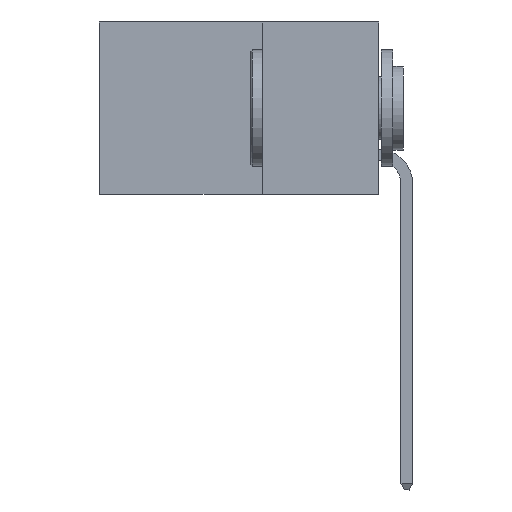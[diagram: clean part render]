
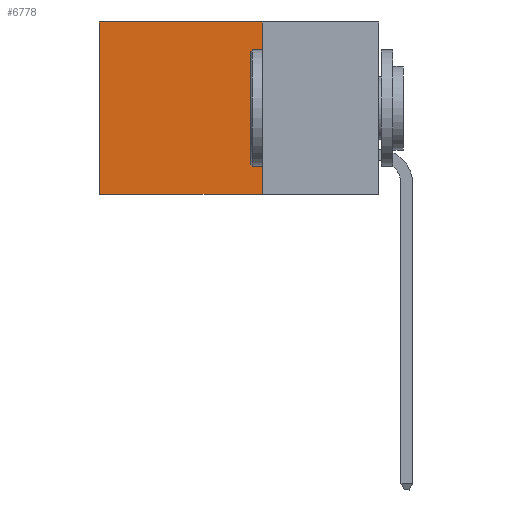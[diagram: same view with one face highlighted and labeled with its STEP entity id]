
A CAD part, left-side view. The second image highlights one B-rep face of the part: STEP entity #6778.
In plain terms, the highlighted planar face has unit normal (-1, 0, 0).
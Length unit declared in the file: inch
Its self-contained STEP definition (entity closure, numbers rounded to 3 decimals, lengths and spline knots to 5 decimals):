
#124 = LINE ( 'NONE', #7433, #5244 ) ;
#285 = VERTEX_POINT ( 'NONE', #12452 ) ;
#310 = CARTESIAN_POINT ( 'NONE',  ( 0.298, 0.25, -0.37 ) ) ;
#1391 = FACE_OUTER_BOUND ( 'NONE', #8691, .T. ) ;
#1457 = CARTESIAN_POINT ( 'NONE',  ( 0.298, 0.25, -0.37 ) ) ;
#1595 = AXIS2_PLACEMENT_3D ( 'NONE', #2496, #4688, #5790 ) ;
#1992 = DIRECTION ( 'NONE',  ( 0., 0., -1. ) ) ;
#2415 = LINE ( 'NONE', #6029, #4167 ) ;
#2431 = VECTOR ( 'NONE', #2647, 39.37008 ) ;
#2496 = CARTESIAN_POINT ( 'NONE',  ( 0.298, 0.25, 0. ) ) ;
#2647 = DIRECTION ( 'NONE',  ( 0., 0., -1. ) ) ;
#3069 = CARTESIAN_POINT ( 'NONE',  ( 0.298, 0.6, 0. ) ) ;
#3127 = ORIENTED_EDGE ( 'NONE', *, *, #12141, .T. ) ;
#4167 = VECTOR ( 'NONE', #10453, 39.37008 ) ;
#4688 = DIRECTION ( 'NONE',  ( 1., 0., 0. ) ) ;
#5244 = VECTOR ( 'NONE', #1992, 39.37008 ) ;
#5340 = LINE ( 'NONE', #9209, #2431 ) ;
#5790 = DIRECTION ( 'NONE',  ( 0., 0., -1. ) ) ;
#6029 = CARTESIAN_POINT ( 'NONE',  ( 0.298, 0.25, 0. ) ) ;
#6320 = VECTOR ( 'NONE', #6954, 39.37008 ) ;
#6778 = ADVANCED_FACE ( 'NONE', ( #1391 ), #12286, .F. ) ;
#6855 = EDGE_CURVE ( 'NONE', #7205, #9113, #2415, .T. ) ;
#6857 = EDGE_CURVE ( 'NONE', #7205, #12838, #5340, .T. ) ;
#6954 = DIRECTION ( 'NONE',  ( 0., 1., 0. ) ) ;
#6963 = ORIENTED_EDGE ( 'NONE', *, *, #6855, .T. ) ;
#7205 = VERTEX_POINT ( 'NONE', #11571 ) ;
#7433 = CARTESIAN_POINT ( 'NONE',  ( 0.298, 0.6, 0. ) ) ;
#8153 = ORIENTED_EDGE ( 'NONE', *, *, #6857, .F. ) ;
#8691 = EDGE_LOOP ( 'NONE', ( #3127, #9604, #8153, #6963 ) ) ;
#9113 = VERTEX_POINT ( 'NONE', #3069 ) ;
#9209 = CARTESIAN_POINT ( 'NONE',  ( 0.298, 0.25, 0. ) ) ;
#9604 = ORIENTED_EDGE ( 'NONE', *, *, #11368, .F. ) ;
#10453 = DIRECTION ( 'NONE',  ( 0., 1., 0. ) ) ;
#11368 = EDGE_CURVE ( 'NONE', #12838, #285, #14170, .T. ) ;
#11571 = CARTESIAN_POINT ( 'NONE',  ( 0.298, 0.25, 0. ) ) ;
#12141 = EDGE_CURVE ( 'NONE', #9113, #285, #124, .T. ) ;
#12286 = PLANE ( 'NONE',  #1595 ) ;
#12452 = CARTESIAN_POINT ( 'NONE',  ( 0.298, 0.6, -0.37 ) ) ;
#12838 = VERTEX_POINT ( 'NONE', #310 ) ;
#14170 = LINE ( 'NONE', #1457, #6320 ) ;
